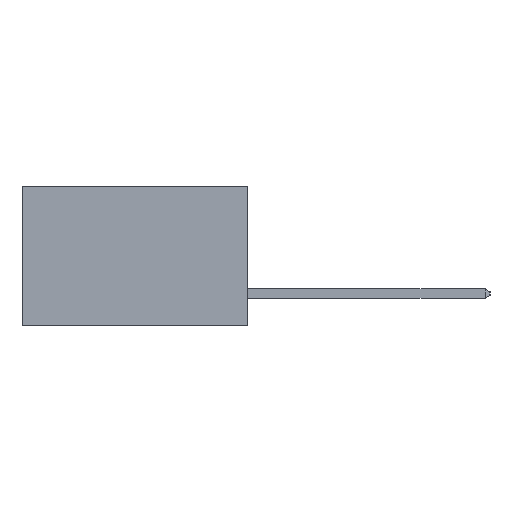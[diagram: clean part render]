
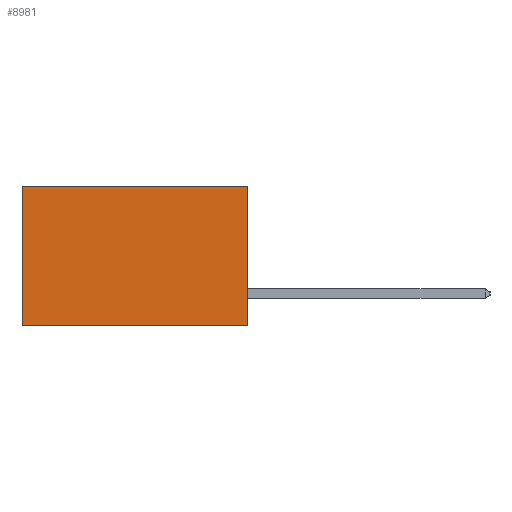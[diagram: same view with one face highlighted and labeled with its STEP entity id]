
A CAD part, left-side view. The second image highlights one B-rep face of the part: STEP entity #8981.
In plain terms, the highlighted planar face has unit normal (-1, 0, 0).
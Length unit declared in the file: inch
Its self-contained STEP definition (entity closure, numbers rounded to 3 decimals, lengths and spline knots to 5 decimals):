
#505 = EDGE_CURVE ( 'NONE', #3973, #3987, #12378, .T. ) ;
#1275 = EDGE_CURVE ( 'NONE', #12976, #3015, #8220, .T. ) ;
#1389 = DIRECTION ( 'NONE',  ( 0., 0., -1. ) ) ;
#1431 = DIRECTION ( 'NONE',  ( 0., 1., 0. ) ) ;
#1443 = CARTESIAN_POINT ( 'NONE',  ( 0.2615, 0.6, -0.37 ) ) ;
#2319 = DIRECTION ( 'NONE',  ( 0., 1., 0. ) ) ;
#2446 = CARTESIAN_POINT ( 'NONE',  ( 0.2615, 0., 0. ) ) ;
#2505 = DIRECTION ( 'NONE',  ( 0., 0., -1. ) ) ;
#2519 = VECTOR ( 'NONE', #2319, 39.37008 ) ;
#3015 = VERTEX_POINT ( 'NONE', #13870 ) ;
#3103 = ORIENTED_EDGE ( 'NONE', *, *, #4378, .T. ) ;
#3973 = VERTEX_POINT ( 'NONE', #10259 ) ;
#3987 = VERTEX_POINT ( 'NONE', #4501 ) ;
#4378 = EDGE_CURVE ( 'NONE', #12976, #3973, #5730, .T. ) ;
#4501 = CARTESIAN_POINT ( 'NONE',  ( 0.2615, 0.6, -0.37 ) ) ;
#5593 = EDGE_CURVE ( 'NONE', #3015, #3987, #6078, .T. ) ;
#5730 = LINE ( 'NONE', #2446, #2519 ) ;
#5787 = CARTESIAN_POINT ( 'NONE',  ( 0.2615, 0., -0.37 ) ) ;
#6078 = LINE ( 'NONE', #8623, #6472 ) ;
#6472 = VECTOR ( 'NONE', #1431, 39.37008 ) ;
#7400 = CARTESIAN_POINT ( 'NONE',  ( 0.2615, 0., 0. ) ) ;
#7565 = DIRECTION ( 'NONE',  ( 0., 0., -1. ) ) ;
#7841 = FACE_OUTER_BOUND ( 'NONE', #9665, .T. ) ;
#8220 = LINE ( 'NONE', #5787, #15086 ) ;
#8623 = CARTESIAN_POINT ( 'NONE',  ( 0.2615, 0., -0.37 ) ) ;
#8658 = ORIENTED_EDGE ( 'NONE', *, *, #505, .T. ) ;
#8804 = VECTOR ( 'NONE', #1389, 39.37008 ) ;
#8958 = AXIS2_PLACEMENT_3D ( 'NONE', #13599, #14855, #7565 ) ;
#8981 = ADVANCED_FACE ( 'NONE', ( #7841 ), #12341, .F. ) ;
#9665 = EDGE_LOOP ( 'NONE', ( #8658, #10531, #13294, #3103 ) ) ;
#10259 = CARTESIAN_POINT ( 'NONE',  ( 0.2615, 0.6, 0. ) ) ;
#10531 = ORIENTED_EDGE ( 'NONE', *, *, #5593, .F. ) ;
#12341 = PLANE ( 'NONE',  #8958 ) ;
#12378 = LINE ( 'NONE', #1443, #8804 ) ;
#12976 = VERTEX_POINT ( 'NONE', #7400 ) ;
#13294 = ORIENTED_EDGE ( 'NONE', *, *, #1275, .F. ) ;
#13599 = CARTESIAN_POINT ( 'NONE',  ( 0.2615, 0., -0.37 ) ) ;
#13870 = CARTESIAN_POINT ( 'NONE',  ( 0.2615, 0., -0.37 ) ) ;
#14855 = DIRECTION ( 'NONE',  ( 1., 0., 0. ) ) ;
#15086 = VECTOR ( 'NONE', #2505, 39.37008 ) ;
